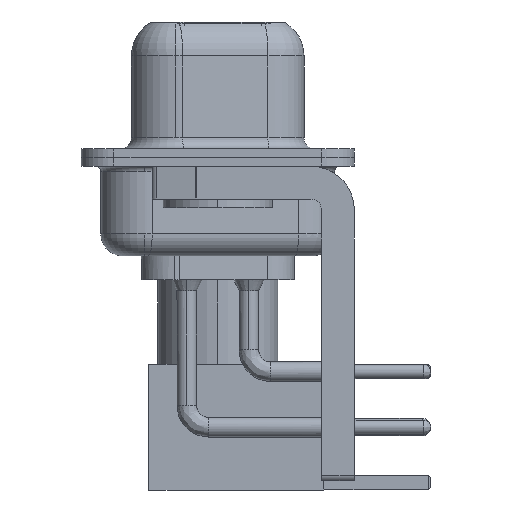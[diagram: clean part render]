
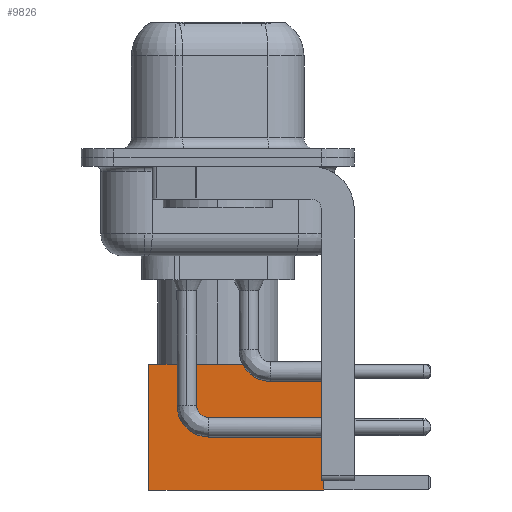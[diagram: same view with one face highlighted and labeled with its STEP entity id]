
A CAD part, left-side view. The second image highlights one B-rep face of the part: STEP entity #9826.
In plain terms, the highlighted face is planar.
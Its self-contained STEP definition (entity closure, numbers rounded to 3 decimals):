
#2266 = CARTESIAN_POINT ( 'NONE',  ( 0., 2.875, 8. ) ) ;
#2610 = ORIENTED_EDGE ( 'NONE', *, *, #15066, .F. ) ;
#2862 = CARTESIAN_POINT ( 'NONE',  ( 2.875, 2.875, 0. ) ) ;
#4336 = DIRECTION ( 'NONE',  ( 0., 0., -1. ) ) ;
#4846 = VERTEX_POINT ( 'NONE', #9402 ) ;
#4933 = CARTESIAN_POINT ( 'NONE',  ( 2.875, 2.875, 0. ) ) ;
#4969 = VECTOR ( 'NONE', #18966, 1000. ) ;
#4976 = LINE ( 'NONE', #13790, #4969 ) ;
#5872 = ORIENTED_EDGE ( 'NONE', *, *, #15344, .F. ) ;
#6060 = PLANE ( 'NONE',  #14862 ) ;
#6250 = EDGE_CURVE ( 'NONE', #16343, #16965, #4976, .T. ) ;
#6422 = ORIENTED_EDGE ( 'NONE', *, *, #6250, .T. ) ;
#7771 = LINE ( 'NONE', #14769, #14600 ) ;
#9402 = CARTESIAN_POINT ( 'NONE',  ( -2.875, 2.875, 8. ) ) ;
#9826 = ADVANCED_FACE ( 'NONE', ( #14657 ), #6060, .T. ) ;
#11316 = DIRECTION ( 'NONE',  ( -1., 0., 0. ) ) ;
#11449 = VERTEX_POINT ( 'NONE', #19036 ) ;
#12565 = LINE ( 'NONE', #2266, #18656 ) ;
#13041 = CARTESIAN_POINT ( 'NONE',  ( 0., 2.875, 0. ) ) ;
#13301 = VECTOR ( 'NONE', #11316, 1000. ) ;
#13790 = CARTESIAN_POINT ( 'NONE',  ( 2.875, 2.875, 0. ) ) ;
#14514 = DIRECTION ( 'NONE',  ( -1., 0., 0. ) ) ;
#14538 = LINE ( 'NONE', #13041, #13301 ) ;
#14600 = VECTOR ( 'NONE', #4336, 1000. ) ;
#14657 = FACE_OUTER_BOUND ( 'NONE', #18433, .T. ) ;
#14769 = CARTESIAN_POINT ( 'NONE',  ( -2.875, 2.875, 0. ) ) ;
#14862 = AXIS2_PLACEMENT_3D ( 'NONE', #2862, #19926, #15110 ) ;
#15066 = EDGE_CURVE ( 'NONE', #4846, #11449, #7771, .T. ) ;
#15110 = DIRECTION ( 'NONE',  ( 0., 0., 1. ) ) ;
#15344 = EDGE_CURVE ( 'NONE', #16343, #4846, #12565, .T. ) ;
#16343 = VERTEX_POINT ( 'NONE', #18503 ) ;
#16965 = VERTEX_POINT ( 'NONE', #4933 ) ;
#18433 = EDGE_LOOP ( 'NONE', ( #6422, #19598, #2610, #5872 ) ) ;
#18503 = CARTESIAN_POINT ( 'NONE',  ( 2.875, 2.875, 8. ) ) ;
#18656 = VECTOR ( 'NONE', #14514, 1000. ) ;
#18966 = DIRECTION ( 'NONE',  ( 0., 0., -1. ) ) ;
#19036 = CARTESIAN_POINT ( 'NONE',  ( -2.875, 2.875, 0. ) ) ;
#19350 = EDGE_CURVE ( 'NONE', #16965, #11449, #14538, .T. ) ;
#19598 = ORIENTED_EDGE ( 'NONE', *, *, #19350, .T. ) ;
#19926 = DIRECTION ( 'NONE',  ( 0., 1., 0. ) ) ;
